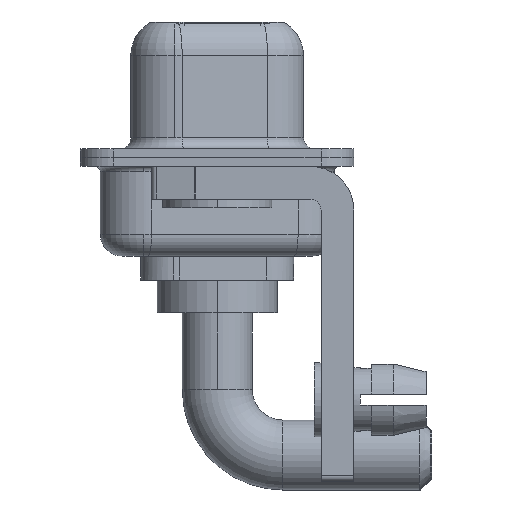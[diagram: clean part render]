
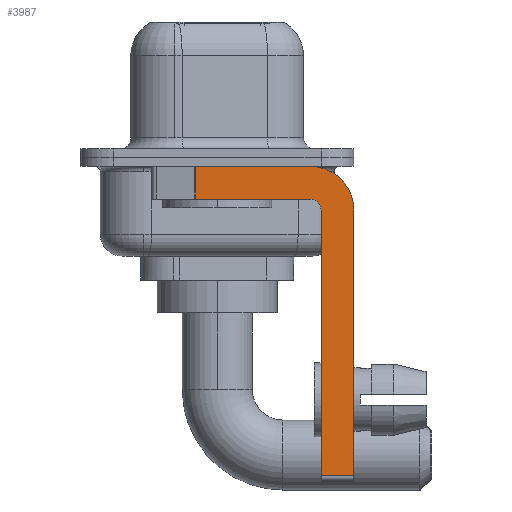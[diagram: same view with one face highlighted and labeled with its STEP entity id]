
A CAD part, left-side view. The second image highlights one B-rep face of the part: STEP entity #3987.
In plain terms, the highlighted planar face has unit normal (-1, 0, 0).
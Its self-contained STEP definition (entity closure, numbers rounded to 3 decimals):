
#13 = CARTESIAN_POINT ( 'NONE',  ( -2.9, -4.25, -0.4 ) ) ;
#221 = EDGE_CURVE ( 'NONE', #9701, #5673, #1944, .T. ) ;
#273 = VERTEX_POINT ( 'NONE', #11528 ) ;
#276 = CARTESIAN_POINT ( 'NONE',  ( -2.9, 0.978, -1.9 ) ) ;
#317 = ORIENTED_EDGE ( 'NONE', *, *, #10052, .F. ) ;
#1013 = VECTOR ( 'NONE', #8136, 1000. ) ;
#1088 = VERTEX_POINT ( 'NONE', #276 ) ;
#1113 = CARTESIAN_POINT ( 'NONE',  ( -2.9, -6.25, -2.4 ) ) ;
#1156 = VECTOR ( 'NONE', #11521, 1000. ) ;
#1415 = VERTEX_POINT ( 'NONE', #7178 ) ;
#1944 = CIRCLE ( 'NONE', #14136, 2. ) ;
#1997 = LINE ( 'NONE', #11696, #3791 ) ;
#2013 = LINE ( 'NONE', #14259, #1013 ) ;
#2076 = DIRECTION ( 'NONE',  ( 0., 0., 1. ) ) ;
#2247 = DIRECTION ( 'NONE',  ( 1., 0., 0. ) ) ;
#2667 = DIRECTION ( 'NONE',  ( 0., -1., 0. ) ) ;
#3258 = DIRECTION ( 'NONE',  ( -1., 0., 0. ) ) ;
#3316 = ORIENTED_EDGE ( 'NONE', *, *, #4484, .F. ) ;
#3322 = VERTEX_POINT ( 'NONE', #13833 ) ;
#3577 = EDGE_LOOP ( 'NONE', ( #3754, #13056, #317, #8367, #3316, #4387, #4499, #14598 ) ) ;
#3619 = EDGE_CURVE ( 'NONE', #3322, #11191, #9991, .T. ) ;
#3754 = ORIENTED_EDGE ( 'NONE', *, *, #12525, .F. ) ;
#3783 = AXIS2_PLACEMENT_3D ( 'NONE', #8232, #2247, #5914 ) ;
#3791 = VECTOR ( 'NONE', #10519, 1000. ) ;
#3982 = CARTESIAN_POINT ( 'NONE',  ( -2.9, -4.25, -2.4 ) ) ;
#3987 = ADVANCED_FACE ( 'NONE', ( #10620 ), #10703, .F. ) ;
#4128 = CARTESIAN_POINT ( 'NONE',  ( -2.9, 0.978, -0.4 ) ) ;
#4387 = ORIENTED_EDGE ( 'NONE', *, *, #3619, .T. ) ;
#4484 = EDGE_CURVE ( 'NONE', #3322, #273, #1997, .T. ) ;
#4487 = EDGE_CURVE ( 'NONE', #273, #1415, #14210, .T. ) ;
#4499 = ORIENTED_EDGE ( 'NONE', *, *, #15189, .F. ) ;
#5484 = CARTESIAN_POINT ( 'NONE',  ( -2.9, -4.25, -1.9 ) ) ;
#5673 = VERTEX_POINT ( 'NONE', #14682 ) ;
#5864 = LINE ( 'NONE', #10736, #11447 ) ;
#5914 = DIRECTION ( 'NONE',  ( 0., 0., -1. ) ) ;
#7178 = CARTESIAN_POINT ( 'NONE',  ( -2.9, -4.25, -1.9 ) ) ;
#7580 = VECTOR ( 'NONE', #2667, 1000. ) ;
#8136 = DIRECTION ( 'NONE',  ( 0., 0., -1. ) ) ;
#8232 = CARTESIAN_POINT ( 'NONE',  ( -2.9, -4.25, -2.4 ) ) ;
#8367 = ORIENTED_EDGE ( 'NONE', *, *, #4487, .F. ) ;
#8434 = DIRECTION ( 'NONE',  ( 0., 0., -1. ) ) ;
#8646 = VERTEX_POINT ( 'NONE', #4128 ) ;
#8838 = DIRECTION ( 'NONE',  ( 1., 0., 0. ) ) ;
#9002 = DIRECTION ( 'NONE',  ( 0., 0., -1. ) ) ;
#9701 = VERTEX_POINT ( 'NONE', #13 ) ;
#9991 = LINE ( 'NONE', #13556, #7580 ) ;
#10052 = EDGE_CURVE ( 'NONE', #1415, #1088, #15108, .T. ) ;
#10234 = VECTOR ( 'NONE', #8434, 1000. ) ;
#10519 = DIRECTION ( 'NONE',  ( 0., 0., 1. ) ) ;
#10620 = FACE_OUTER_BOUND ( 'NONE', #3577, .T. ) ;
#10703 = PLANE ( 'NONE',  #3783 ) ;
#10736 = CARTESIAN_POINT ( 'NONE',  ( -2.9, 3., -0.4 ) ) ;
#10975 = EDGE_CURVE ( 'NONE', #8646, #1088, #2013, .T. ) ;
#11191 = VERTEX_POINT ( 'NONE', #14573 ) ;
#11447 = VECTOR ( 'NONE', #14383, 1000. ) ;
#11521 = DIRECTION ( 'NONE',  ( 0., 1., 0. ) ) ;
#11528 = CARTESIAN_POINT ( 'NONE',  ( -2.9, -4.75, -2.4 ) ) ;
#11696 = CARTESIAN_POINT ( 'NONE',  ( -2.9, -4.75, -14.8 ) ) ;
#11782 = LINE ( 'NONE', #1113, #10234 ) ;
#12525 = EDGE_CURVE ( 'NONE', #8646, #9701, #5864, .T. ) ;
#12685 = AXIS2_PLACEMENT_3D ( 'NONE', #15359, #3258, #2076 ) ;
#13056 = ORIENTED_EDGE ( 'NONE', *, *, #10975, .T. ) ;
#13556 = CARTESIAN_POINT ( 'NONE',  ( -2.9, -4.25, -14.55 ) ) ;
#13833 = CARTESIAN_POINT ( 'NONE',  ( -2.9, -4.75, -14.55 ) ) ;
#14136 = AXIS2_PLACEMENT_3D ( 'NONE', #3982, #8838, #9002 ) ;
#14210 = CIRCLE ( 'NONE', #12685, 0.5 ) ;
#14259 = CARTESIAN_POINT ( 'NONE',  ( -2.9, 0.978, -1.9 ) ) ;
#14383 = DIRECTION ( 'NONE',  ( 0., -1., 0. ) ) ;
#14573 = CARTESIAN_POINT ( 'NONE',  ( -2.9, -6.25, -14.55 ) ) ;
#14598 = ORIENTED_EDGE ( 'NONE', *, *, #221, .F. ) ;
#14682 = CARTESIAN_POINT ( 'NONE',  ( -2.9, -6.25, -2.4 ) ) ;
#15108 = LINE ( 'NONE', #5484, #1156 ) ;
#15189 = EDGE_CURVE ( 'NONE', #5673, #11191, #11782, .T. ) ;
#15359 = CARTESIAN_POINT ( 'NONE',  ( -2.9, -4.25, -2.4 ) ) ;
